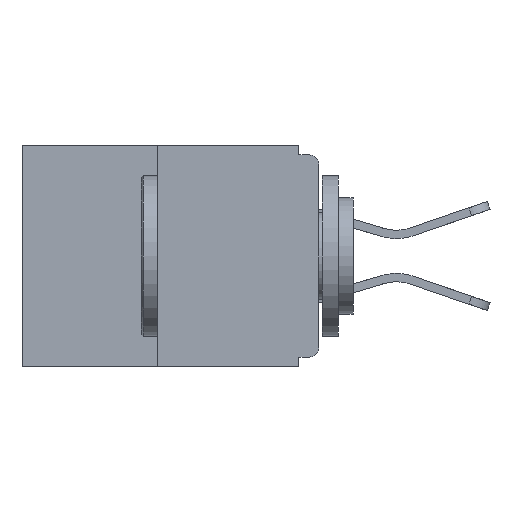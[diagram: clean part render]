
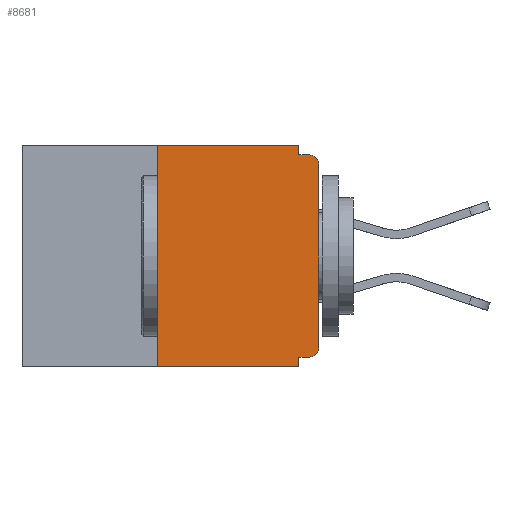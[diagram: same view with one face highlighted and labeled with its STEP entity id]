
A CAD part, left-side view. The second image highlights one B-rep face of the part: STEP entity #8681.
In plain terms, the highlighted planar face has unit normal (-1, 0, 0).
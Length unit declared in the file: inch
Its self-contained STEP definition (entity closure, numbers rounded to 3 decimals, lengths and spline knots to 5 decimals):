
#263 = EDGE_CURVE ( 'NONE', #12430, #12393, #13811, .T. ) ;
#738 = LINE ( 'NONE', #12180, #7864 ) ;
#1036 = EDGE_CURVE ( 'NONE', #6101, #14184, #12329, .T. ) ;
#1070 = EDGE_CURVE ( 'NONE', #2615, #14787, #738, .T. ) ;
#1251 = VERTEX_POINT ( 'NONE', #12676 ) ;
#1598 = CIRCLE ( 'NONE', #7934, 0.015 ) ;
#1684 = DIRECTION ( 'NONE',  ( 0., 1., 0. ) ) ;
#1734 = LINE ( 'NONE', #6016, #3749 ) ;
#2516 = DIRECTION ( 'NONE',  ( 0., -1., 0. ) ) ;
#2534 = DIRECTION ( 'NONE',  ( -1., 0., 0. ) ) ;
#2572 = CARTESIAN_POINT ( 'NONE',  ( 0., 0.031, -0.015 ) ) ;
#2615 = VERTEX_POINT ( 'NONE', #7106 ) ;
#2638 = CARTESIAN_POINT ( 'NONE',  ( 0., 0.031, -0.328 ) ) ;
#2762 = ORIENTED_EDGE ( 'NONE', *, *, #5341, .T. ) ;
#2848 = EDGE_CURVE ( 'NONE', #2615, #10735, #7499, .T. ) ;
#2872 = CARTESIAN_POINT ( 'NONE',  ( 0., 0., -0.328 ) ) ;
#2894 = EDGE_LOOP ( 'NONE', ( #8636, #10779, #9889, #3789, #13537, #7381, #2762, #14338, #10030, #2902 ) ) ;
#2902 = ORIENTED_EDGE ( 'NONE', *, *, #7083, .F. ) ;
#2994 = VECTOR ( 'NONE', #9851, 39.37008 ) ;
#3285 = CARTESIAN_POINT ( 'NONE',  ( 0., 0.015, -0.328 ) ) ;
#3525 = CARTESIAN_POINT ( 'NONE',  ( 0., 0.015, -0.015 ) ) ;
#3698 = CARTESIAN_POINT ( 'NONE',  ( 0., 0.46, 0. ) ) ;
#3749 = VECTOR ( 'NONE', #2516, 39.37008 ) ;
#3767 = VECTOR ( 'NONE', #1684, 39.37008 ) ;
#3789 = ORIENTED_EDGE ( 'NONE', *, *, #5954, .F. ) ;
#4267 = FACE_OUTER_BOUND ( 'NONE', #2894, .T. ) ;
#4627 = AXIS2_PLACEMENT_3D ( 'NONE', #8469, #2534, #14544 ) ;
#4884 = VECTOR ( 'NONE', #11941, 39.37008 ) ;
#5341 = EDGE_CURVE ( 'NONE', #14184, #10986, #6846, .T. ) ;
#5954 = EDGE_CURVE ( 'NONE', #6229, #10735, #14109, .T. ) ;
#5966 = CARTESIAN_POINT ( 'NONE',  ( 0., 0.46, -0.343 ) ) ;
#6016 = CARTESIAN_POINT ( 'NONE',  ( 0., 0.46, 0. ) ) ;
#6055 = DIRECTION ( 'NONE',  ( 1., 0., 0. ) ) ;
#6101 = VERTEX_POINT ( 'NONE', #3285 ) ;
#6167 = DIRECTION ( 'NONE',  ( 0., 0., -1. ) ) ;
#6229 = VERTEX_POINT ( 'NONE', #2638 ) ;
#6846 = LINE ( 'NONE', #11892, #15238 ) ;
#7083 = EDGE_CURVE ( 'NONE', #1251, #12430, #11105, .T. ) ;
#7106 = CARTESIAN_POINT ( 'NONE',  ( 0., 0.25, -0.343 ) ) ;
#7212 = CARTESIAN_POINT ( 'NONE',  ( 0., 0., -0.03 ) ) ;
#7381 = ORIENTED_EDGE ( 'NONE', *, *, #1036, .T. ) ;
#7444 = DIRECTION ( 'NONE',  ( 0., 0., -1. ) ) ;
#7499 = LINE ( 'NONE', #5966, #10146 ) ;
#7817 = DIRECTION ( 'NONE',  ( -1., 0., 0. ) ) ;
#7864 = VECTOR ( 'NONE', #13162, 39.37008 ) ;
#7934 = AXIS2_PLACEMENT_3D ( 'NONE', #11372, #7817, #12449 ) ;
#8469 = CARTESIAN_POINT ( 'NONE',  ( 0., 0.015, -0.313 ) ) ;
#8482 = DIRECTION ( 'NONE',  ( 0., 0., 1. ) ) ;
#8636 = ORIENTED_EDGE ( 'NONE', *, *, #13948, .F. ) ;
#8681 = ADVANCED_FACE ( 'NONE', ( #4267 ), #13178, .F. ) ;
#9050 = CARTESIAN_POINT ( 'NONE',  ( 0., 0.031, -0.343 ) ) ;
#9492 = CARTESIAN_POINT ( 'NONE',  ( 0., 0.031, 0. ) ) ;
#9851 = DIRECTION ( 'NONE',  ( 0., -1., 0. ) ) ;
#9889 = ORIENTED_EDGE ( 'NONE', *, *, #2848, .T. ) ;
#10030 = ORIENTED_EDGE ( 'NONE', *, *, #263, .F. ) ;
#10146 = VECTOR ( 'NONE', #10598, 39.37008 ) ;
#10181 = LINE ( 'NONE', #2872, #3767 ) ;
#10598 = DIRECTION ( 'NONE',  ( 0., -1., 0. ) ) ;
#10735 = VERTEX_POINT ( 'NONE', #9050 ) ;
#10779 = ORIENTED_EDGE ( 'NONE', *, *, #1070, .F. ) ;
#10953 = VECTOR ( 'NONE', #7444, 39.37008 ) ;
#10986 = VERTEX_POINT ( 'NONE', #7212 ) ;
#10987 = CARTESIAN_POINT ( 'NONE',  ( 0., 0., -0.015 ) ) ;
#11004 = CARTESIAN_POINT ( 'NONE',  ( 0., 0.031, -0.343 ) ) ;
#11105 = LINE ( 'NONE', #9492, #4884 ) ;
#11372 = CARTESIAN_POINT ( 'NONE',  ( 0., 0.015, -0.03 ) ) ;
#11601 = CARTESIAN_POINT ( 'NONE',  ( 0., 0.25, 0. ) ) ;
#11892 = CARTESIAN_POINT ( 'NONE',  ( 0., 0., 0. ) ) ;
#11941 = DIRECTION ( 'NONE',  ( 0., 0., -1. ) ) ;
#12006 = EDGE_CURVE ( 'NONE', #10986, #12393, #1598, .T. ) ;
#12180 = CARTESIAN_POINT ( 'NONE',  ( 0., 0.25, 0. ) ) ;
#12329 = CIRCLE ( 'NONE', #4627, 0.015 ) ;
#12393 = VERTEX_POINT ( 'NONE', #3525 ) ;
#12430 = VERTEX_POINT ( 'NONE', #2572 ) ;
#12449 = DIRECTION ( 'NONE',  ( 0., 0., -1. ) ) ;
#12565 = AXIS2_PLACEMENT_3D ( 'NONE', #3698, #6055, #6167 ) ;
#12676 = CARTESIAN_POINT ( 'NONE',  ( 0., 0.031, 0. ) ) ;
#13162 = DIRECTION ( 'NONE',  ( 0., 0., 1. ) ) ;
#13178 = PLANE ( 'NONE',  #12565 ) ;
#13390 = EDGE_CURVE ( 'NONE', #6101, #6229, #10181, .T. ) ;
#13537 = ORIENTED_EDGE ( 'NONE', *, *, #13390, .F. ) ;
#13811 = LINE ( 'NONE', #10987, #2994 ) ;
#13948 = EDGE_CURVE ( 'NONE', #14787, #1251, #1734, .T. ) ;
#14109 = LINE ( 'NONE', #11004, #10953 ) ;
#14184 = VERTEX_POINT ( 'NONE', #15301 ) ;
#14338 = ORIENTED_EDGE ( 'NONE', *, *, #12006, .T. ) ;
#14544 = DIRECTION ( 'NONE',  ( 0., 0., -1. ) ) ;
#14787 = VERTEX_POINT ( 'NONE', #11601 ) ;
#15238 = VECTOR ( 'NONE', #8482, 39.37008 ) ;
#15301 = CARTESIAN_POINT ( 'NONE',  ( 0., 0., -0.313 ) ) ;
